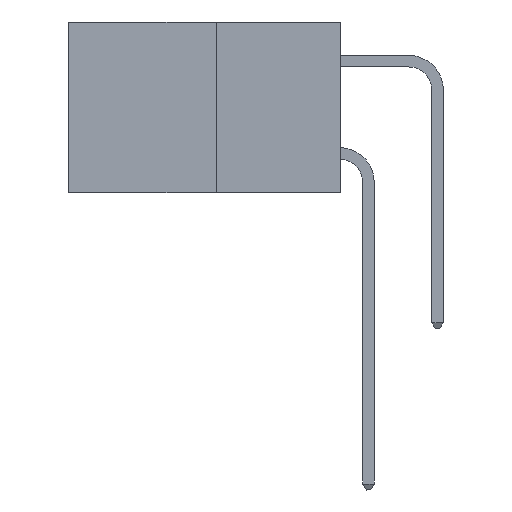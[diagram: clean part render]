
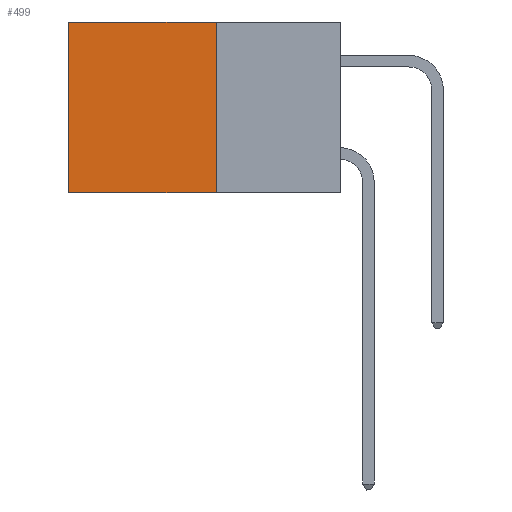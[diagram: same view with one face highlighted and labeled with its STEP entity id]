
A CAD part, left-side view. The second image highlights one B-rep face of the part: STEP entity #499.
In plain terms, the highlighted planar face has unit normal (-1, 0, 0).
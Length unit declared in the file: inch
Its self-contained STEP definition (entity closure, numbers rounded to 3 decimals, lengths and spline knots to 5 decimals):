
#219 = VERTEX_POINT ( 'NONE', #7094 ) ;
#499 = ADVANCED_FACE ( 'NONE', ( #9525 ), #8430, .F. ) ;
#812 = VECTOR ( 'NONE', #4900, 39.37008 ) ;
#873 = AXIS2_PLACEMENT_3D ( 'NONE', #1879, #10731, #7152 ) ;
#894 = ORIENTED_EDGE ( 'NONE', *, *, #2129, .F. ) ;
#1149 = LINE ( 'NONE', #4922, #812 ) ;
#1190 = CARTESIAN_POINT ( 'NONE',  ( 0.277, 0.27, -0.37 ) ) ;
#1422 = EDGE_CURVE ( 'NONE', #219, #4316, #7104, .T. ) ;
#1535 = ORIENTED_EDGE ( 'NONE', *, *, #5382, .F. ) ;
#1635 = ORIENTED_EDGE ( 'NONE', *, *, #1422, .T. ) ;
#1748 = CARTESIAN_POINT ( 'NONE',  ( 0.277, 0.27, -0.37 ) ) ;
#1804 = EDGE_CURVE ( 'NONE', #4316, #5253, #8630, .T. ) ;
#1879 = CARTESIAN_POINT ( 'NONE',  ( 0.277, 0.27, -0.37 ) ) ;
#2129 = EDGE_CURVE ( 'NONE', #219, #10015, #5394, .T. ) ;
#4200 = CARTESIAN_POINT ( 'NONE',  ( 0.277, 0.59, -0.37 ) ) ;
#4316 = VERTEX_POINT ( 'NONE', #10606 ) ;
#4825 = EDGE_LOOP ( 'NONE', ( #9033, #1535, #894, #1635 ) ) ;
#4900 = DIRECTION ( 'NONE',  ( 0., 1., 0. ) ) ;
#4922 = CARTESIAN_POINT ( 'NONE',  ( 0.277, 0.27, -0.37 ) ) ;
#5253 = VERTEX_POINT ( 'NONE', #6404 ) ;
#5382 = EDGE_CURVE ( 'NONE', #10015, #5253, #1149, .T. ) ;
#5394 = LINE ( 'NONE', #1190, #7509 ) ;
#6404 = CARTESIAN_POINT ( 'NONE',  ( 0.277, 0.59, -0.37 ) ) ;
#7094 = CARTESIAN_POINT ( 'NONE',  ( 0.277, 0.27, 0. ) ) ;
#7104 = LINE ( 'NONE', #9826, #9204 ) ;
#7152 = DIRECTION ( 'NONE',  ( 0., 0., -1. ) ) ;
#7509 = VECTOR ( 'NONE', #9813, 39.37008 ) ;
#8430 = PLANE ( 'NONE',  #873 ) ;
#8630 = LINE ( 'NONE', #4200, #10692 ) ;
#9033 = ORIENTED_EDGE ( 'NONE', *, *, #1804, .T. ) ;
#9204 = VECTOR ( 'NONE', #9484, 39.37008 ) ;
#9484 = DIRECTION ( 'NONE',  ( 0., 1., 0. ) ) ;
#9525 = FACE_OUTER_BOUND ( 'NONE', #4825, .T. ) ;
#9813 = DIRECTION ( 'NONE',  ( 0., 0., -1. ) ) ;
#9826 = CARTESIAN_POINT ( 'NONE',  ( 0.277, 0.27, 0. ) ) ;
#10015 = VERTEX_POINT ( 'NONE', #1748 ) ;
#10604 = DIRECTION ( 'NONE',  ( 0., 0., -1. ) ) ;
#10606 = CARTESIAN_POINT ( 'NONE',  ( 0.277, 0.59, 0. ) ) ;
#10692 = VECTOR ( 'NONE', #10604, 39.37008 ) ;
#10731 = DIRECTION ( 'NONE',  ( 1., 0., 0. ) ) ;
